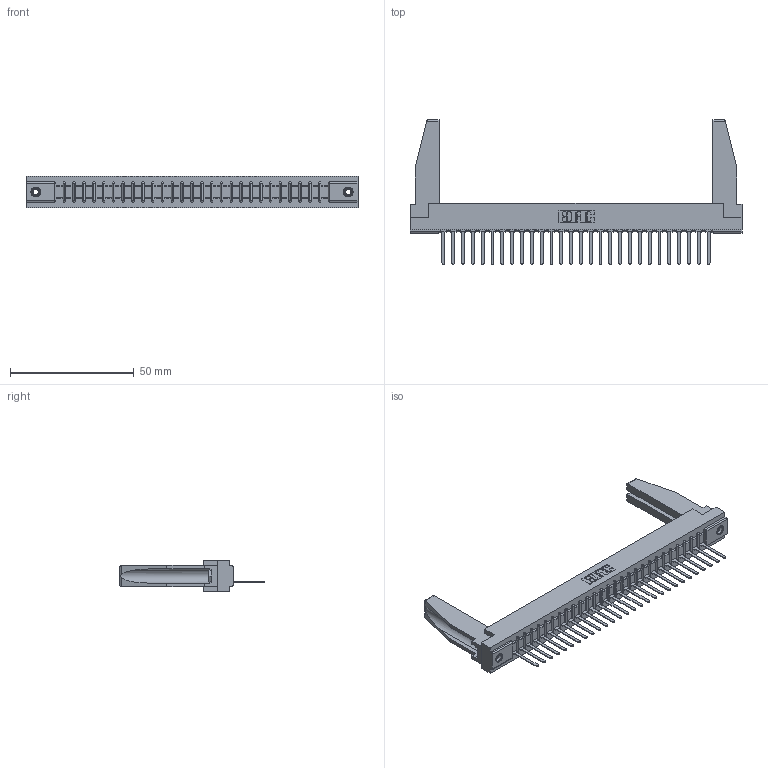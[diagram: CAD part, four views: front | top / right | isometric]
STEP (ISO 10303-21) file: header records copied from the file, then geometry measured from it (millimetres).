
FILE_DESCRIPTION (( 'STEP AP203' ), '1' );
FILE_NAME ('307-028-541-178.STEP', '2019-09-05T03:09:10', ( '' ), ( '' ), 'SwSTEP 2.0', 'SolidWorks 2016', '' );
FILE_SCHEMA (( 'CONFIG_CONTROL_DESIGN' ));
Length unit declared in the file: inch
Products named in the file (5): 307-290-002_541; 307-028-541-178; 307 Part_.156 Dia Mounting Holes; 307-220-078; 345-250-001_345-250-001-102
Assembly tree (33 placements, depth 2):
  307-028-541-178
    307 Part_.156 Dia Mounting Holes
    307-290-002_541  x28
    307-220-078  x2
    345-250-001_345-250-001-102  x2
Bounding box: 133.96 x 58.29 x 12.7 mm (x, y, z)
Volume: 18303.3 mm3; surface area: 22020.2 mm2
Topology: 33 solids, 33 shells, 2349 faces, 7149 edges, 4678 vertices
Faces by surface type: plane 1414, cylinder 861, sphere 58, cone 12, torus 4
Entity records: 28887 total; most frequent: CARTESIAN_POINT 4870, ORIENTED_EDGE 4816, DIRECTION 4694, EDGE_CURVE 2408, VECTOR 1842, LINE 1842, VERTEX_POINT 1560, AXIS2_PLACEMENT_3D 1426
